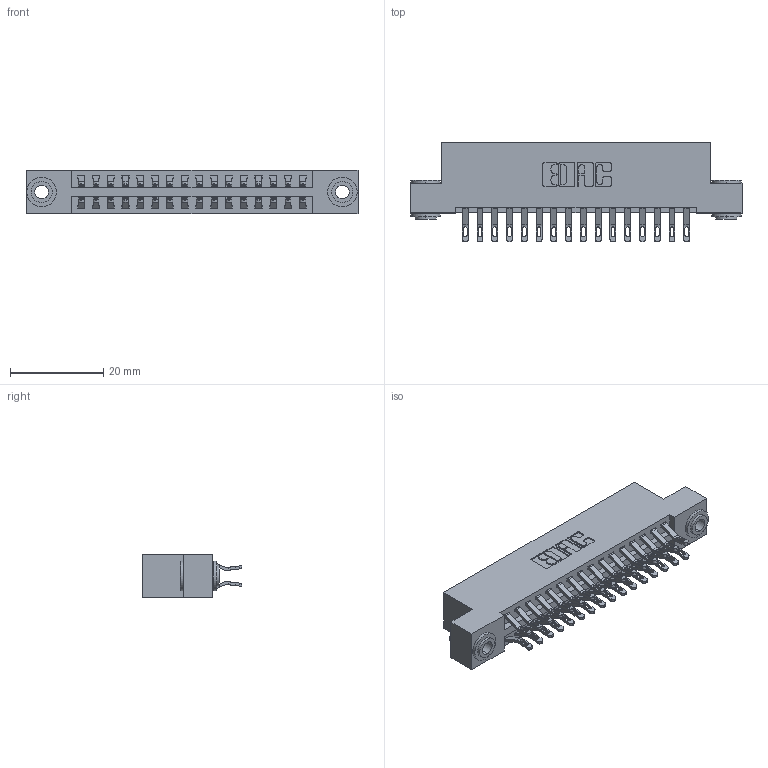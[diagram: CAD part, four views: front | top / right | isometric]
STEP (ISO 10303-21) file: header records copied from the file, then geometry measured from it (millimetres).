
FILE_DESCRIPTION (( 'STEP AP203' ), '1' );
FILE_NAME ('346-032-555-203.STEP', '2022-05-19T18:16:04', ( '' ), ( '' ), 'SwSTEP 2.0', 'SolidWorks 2020', '' );
FILE_SCHEMA (( 'CONFIG_CONTROL_DESIGN' ));
Length unit declared in the file: inch
Products named in the file (4): 345-250-002_345-250-002-102; 345-292-001_555 Tail; 346 Part_Flush Mounting Lugs - 0.156 Dia-TH; 346-032-555-203
Assembly tree (35 placements, depth 2):
  346-032-555-203
    346 Part_Flush Mounting Lugs - 0.156 Dia-TH
    345-292-001_555 Tail  x32
    345-250-002_345-250-002-102  x2
Bounding box: 71.37 x 21.46 x 9.4 mm (x, y, z)
Volume: 6852 mm3; surface area: 9589.5 mm2
Topology: 35 solids, 35 shells, 2030 faces, 6297 edges, 4194 vertices
Faces by surface type: plane 1156, cylinder 866, cone 8
Entity records: 15334 total; most frequent: CARTESIAN_POINT 2579, ORIENTED_EDGE 2474, DIRECTION 2323, EDGE_CURVE 1237, LINE 997, VECTOR 997, VERTEX_POINT 822, AXIS2_PLACEMENT_3D 663
